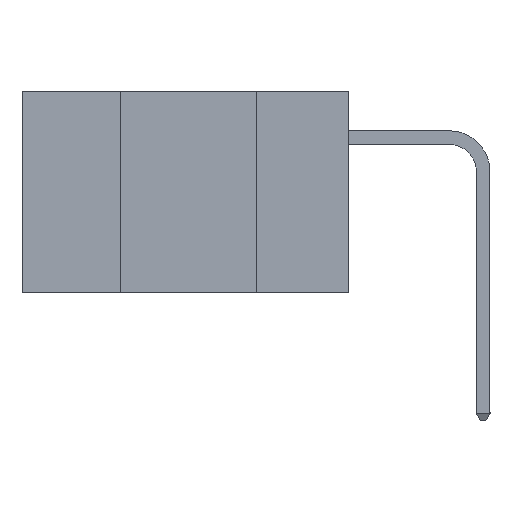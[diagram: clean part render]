
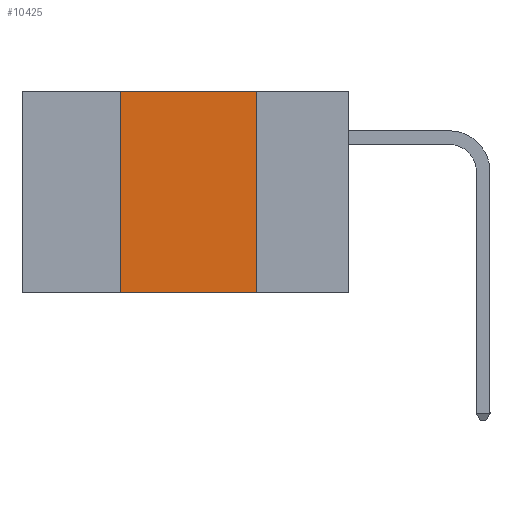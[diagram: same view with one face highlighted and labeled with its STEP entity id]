
A CAD part, left-side view. The second image highlights one B-rep face of the part: STEP entity #10425.
In plain terms, the highlighted planar face has unit normal (-1, 0, 0).
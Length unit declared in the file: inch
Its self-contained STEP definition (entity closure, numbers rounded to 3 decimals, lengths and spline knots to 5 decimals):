
#863 = EDGE_CURVE ( 'NONE', #35526, #10242, #35548, .T. ) ;
#1203 = ORIENTED_EDGE ( 'NONE', *, *, #30541, .F. ) ;
#1500 = CARTESIAN_POINT ( 'NONE',  ( 0., 0.6, -0.37 ) ) ;
#1621 = CARTESIAN_POINT ( 'NONE',  ( 0., 0.17, -0.37 ) ) ;
#2158 = EDGE_CURVE ( 'NONE', #19793, #10242, #4351, .T. ) ;
#3301 = CARTESIAN_POINT ( 'NONE',  ( 0., 0.42, 0. ) ) ;
#3325 = DIRECTION ( 'NONE',  ( 0., 0., -1. ) ) ;
#4351 = LINE ( 'NONE', #1500, #30697 ) ;
#5176 = DIRECTION ( 'NONE',  ( 0., -1., 0. ) ) ;
#5603 = VECTOR ( 'NONE', #26650, 39.37008 ) ;
#6256 = AXIS2_PLACEMENT_3D ( 'NONE', #23597, #23201, #3325 ) ;
#6350 = DIRECTION ( 'NONE',  ( 0., -1., 0. ) ) ;
#8545 = CARTESIAN_POINT ( 'NONE',  ( 0., 0.6, 0. ) ) ;
#9212 = LINE ( 'NONE', #3301, #5603 ) ;
#10242 = VERTEX_POINT ( 'NONE', #1621 ) ;
#10425 = ADVANCED_FACE ( 'NONE', ( #20142 ), #17077, .F. ) ;
#14995 = ORIENTED_EDGE ( 'NONE', *, *, #30813, .F. ) ;
#15416 = VECTOR ( 'NONE', #5176, 39.37008 ) ;
#15970 = ORIENTED_EDGE ( 'NONE', *, *, #863, .F. ) ;
#17077 = PLANE ( 'NONE',  #6256 ) ;
#17952 = CARTESIAN_POINT ( 'NONE',  ( 0., 0.17, 0. ) ) ;
#19793 = VERTEX_POINT ( 'NONE', #26702 ) ;
#20142 = FACE_OUTER_BOUND ( 'NONE', #23803, .T. ) ;
#20429 = CARTESIAN_POINT ( 'NONE',  ( 0., 0.42, 0. ) ) ;
#23201 = DIRECTION ( 'NONE',  ( 1., 0., 0. ) ) ;
#23597 = CARTESIAN_POINT ( 'NONE',  ( 0., 0.6, 0. ) ) ;
#23803 = EDGE_LOOP ( 'NONE', ( #15970, #14995, #1203, #31567 ) ) ;
#25850 = LINE ( 'NONE', #8545, #15416 ) ;
#26650 = DIRECTION ( 'NONE',  ( 0., 0., 1. ) ) ;
#26702 = CARTESIAN_POINT ( 'NONE',  ( 0., 0.42, -0.37 ) ) ;
#29639 = DIRECTION ( 'NONE',  ( 0., 0., -1. ) ) ;
#30541 = EDGE_CURVE ( 'NONE', #19793, #31952, #9212, .T. ) ;
#30697 = VECTOR ( 'NONE', #6350, 39.37008 ) ;
#30813 = EDGE_CURVE ( 'NONE', #31952, #35526, #25850, .T. ) ;
#31567 = ORIENTED_EDGE ( 'NONE', *, *, #2158, .T. ) ;
#31952 = VERTEX_POINT ( 'NONE', #20429 ) ;
#32810 = CARTESIAN_POINT ( 'NONE',  ( 0., 0.17, 0. ) ) ;
#35526 = VERTEX_POINT ( 'NONE', #32810 ) ;
#35548 = LINE ( 'NONE', #17952, #37059 ) ;
#37059 = VECTOR ( 'NONE', #29639, 39.37008 ) ;
